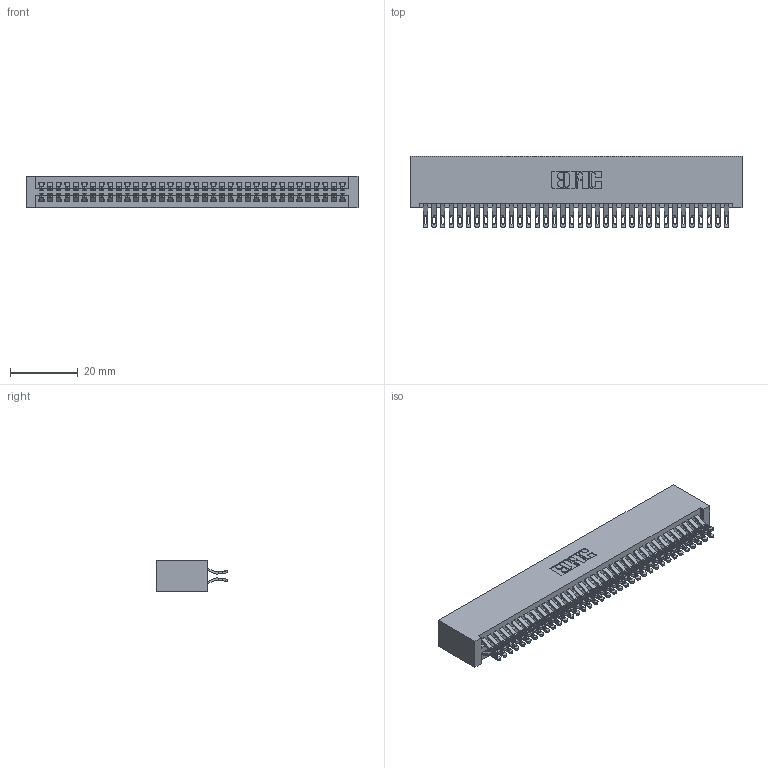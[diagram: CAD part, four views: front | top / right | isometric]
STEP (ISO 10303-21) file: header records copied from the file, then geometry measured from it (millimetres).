
FILE_DESCRIPTION (( 'STEP AP203' ), '1' );
FILE_NAME ('345-072-555-201.STEP', '2018-10-02T08:30:14', ( '' ), ( '' ), 'SwSTEP 2.0', 'SolidWorks 2016', '' );
FILE_SCHEMA (( 'CONFIG_CONTROL_DESIGN' ));
Length unit declared in the file: inch
Products named in the file (3): 345-292-001_555 Tail; 345 Part_No Mounting Lugs; 345-072-555-201
Assembly tree (73 placements, depth 2):
  345-072-555-201
    345 Part_No Mounting Lugs
    345-292-001_555 Tail  x72
Bounding box: 98.04 x 21.13 x 9.4 mm (x, y, z)
Volume: 10293.1 mm3; surface area: 16128.4 mm2
Topology: 73 solids, 73 shells, 4150 faces, 13061 edges, 8706 vertices
Faces by surface type: plane 2308, cylinder 1842
Entity records: 29103 total; most frequent: CARTESIAN_POINT 4918, ORIENTED_EDGE 4822, DIRECTION 4307, EDGE_CURVE 2411, VECTOR 2123, LINE 2123, VERTEX_POINT 1606, AXIS2_PLACEMENT_3D 1092
